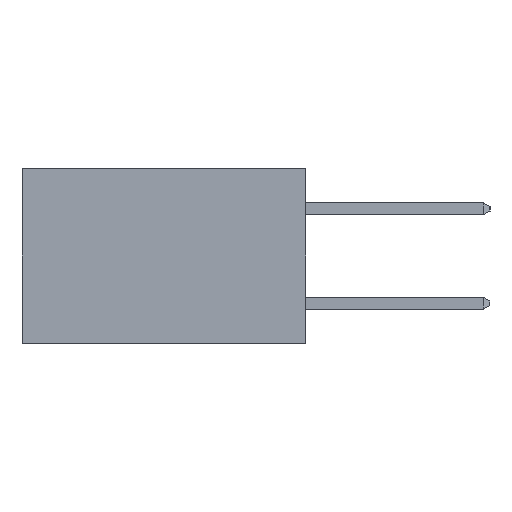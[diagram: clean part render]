
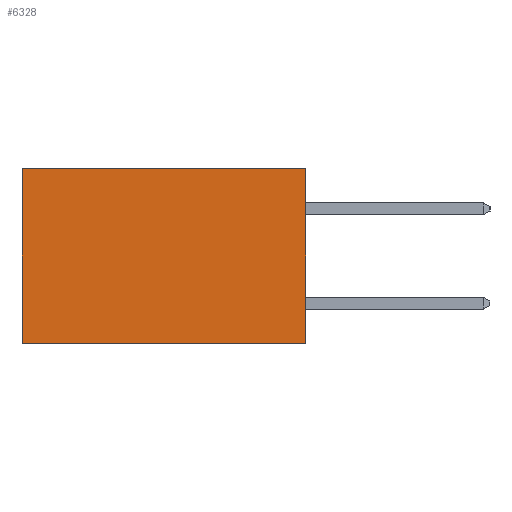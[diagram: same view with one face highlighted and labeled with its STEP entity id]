
A CAD part, left-side view. The second image highlights one B-rep face of the part: STEP entity #6328.
In plain terms, the highlighted planar face has unit normal (-1, 0, 0).
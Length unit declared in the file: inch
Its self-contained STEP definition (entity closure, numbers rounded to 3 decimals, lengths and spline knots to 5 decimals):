
#246 = VECTOR ( 'NONE', #6887, 39.37008 ) ;
#460 = CARTESIAN_POINT ( 'NONE',  ( 0.298, 0., 0. ) ) ;
#507 = DIRECTION ( 'NONE',  ( 0., 0., -1. ) ) ;
#963 = FACE_OUTER_BOUND ( 'NONE', #3951, .T. ) ;
#1190 = CARTESIAN_POINT ( 'NONE',  ( 0.298, 0., 0. ) ) ;
#2074 = VERTEX_POINT ( 'NONE', #1190 ) ;
#2155 = LINE ( 'NONE', #14065, #246 ) ;
#2756 = VERTEX_POINT ( 'NONE', #8900 ) ;
#3951 = EDGE_LOOP ( 'NONE', ( #10088, #6084, #14487, #8455 ) ) ;
#4284 = CARTESIAN_POINT ( 'NONE',  ( 0.298, 0.6, -0.37 ) ) ;
#4358 = EDGE_CURVE ( 'NONE', #8148, #6967, #7745, .T. ) ;
#4437 = VECTOR ( 'NONE', #10741, 39.37008 ) ;
#4443 = VECTOR ( 'NONE', #507, 39.37008 ) ;
#6042 = VECTOR ( 'NONE', #7738, 39.37008 ) ;
#6084 = ORIENTED_EDGE ( 'NONE', *, *, #14726, .F. ) ;
#6328 = ADVANCED_FACE ( 'NONE', ( #963 ), #13261, .F. ) ;
#6455 = CARTESIAN_POINT ( 'NONE',  ( 0.298, 0.6, 0. ) ) ;
#6887 = DIRECTION ( 'NONE',  ( 0., 1., 0. ) ) ;
#6967 = VERTEX_POINT ( 'NONE', #4284 ) ;
#7461 = AXIS2_PLACEMENT_3D ( 'NONE', #12172, #15517, #11154 ) ;
#7520 = CARTESIAN_POINT ( 'NONE',  ( 0.298, 0., 0. ) ) ;
#7738 = DIRECTION ( 'NONE',  ( 0., 1., 0. ) ) ;
#7745 = LINE ( 'NONE', #12291, #4437 ) ;
#8070 = EDGE_CURVE ( 'NONE', #2074, #8148, #9295, .T. ) ;
#8148 = VERTEX_POINT ( 'NONE', #6455 ) ;
#8455 = ORIENTED_EDGE ( 'NONE', *, *, #8070, .T. ) ;
#8900 = CARTESIAN_POINT ( 'NONE',  ( 0.298, 0., -0.37 ) ) ;
#9295 = LINE ( 'NONE', #7520, #6042 ) ;
#9487 = EDGE_CURVE ( 'NONE', #2074, #2756, #10895, .T. ) ;
#10088 = ORIENTED_EDGE ( 'NONE', *, *, #4358, .T. ) ;
#10741 = DIRECTION ( 'NONE',  ( 0., 0., -1. ) ) ;
#10895 = LINE ( 'NONE', #460, #4443 ) ;
#11154 = DIRECTION ( 'NONE',  ( 0., 0., -1. ) ) ;
#12172 = CARTESIAN_POINT ( 'NONE',  ( 0.298, 0., 0. ) ) ;
#12291 = CARTESIAN_POINT ( 'NONE',  ( 0.298, 0.6, 0. ) ) ;
#13261 = PLANE ( 'NONE',  #7461 ) ;
#14065 = CARTESIAN_POINT ( 'NONE',  ( 0.298, 0., -0.37 ) ) ;
#14487 = ORIENTED_EDGE ( 'NONE', *, *, #9487, .F. ) ;
#14726 = EDGE_CURVE ( 'NONE', #2756, #6967, #2155, .T. ) ;
#15517 = DIRECTION ( 'NONE',  ( 1., 0., 0. ) ) ;
